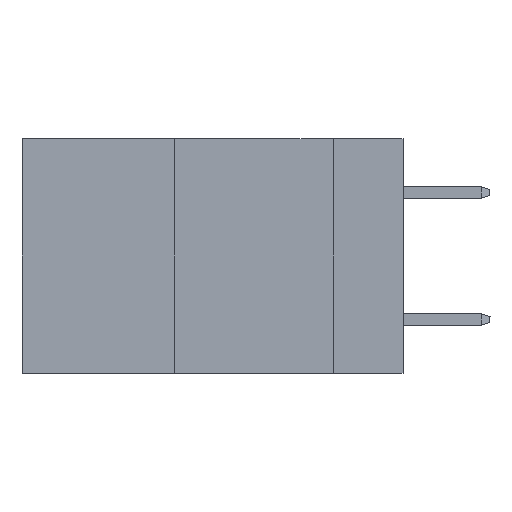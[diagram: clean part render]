
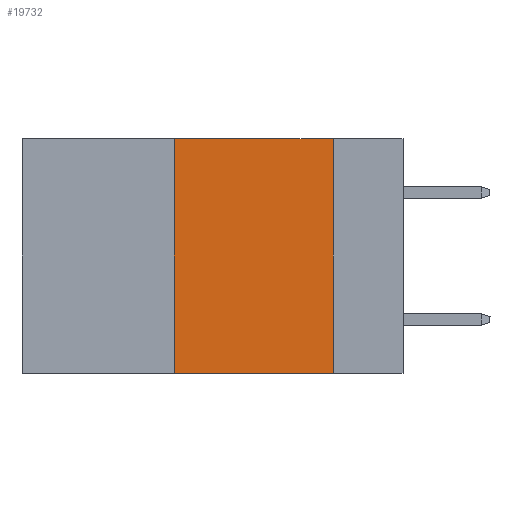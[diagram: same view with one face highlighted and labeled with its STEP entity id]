
A CAD part, left-side view. The second image highlights one B-rep face of the part: STEP entity #19732.
In plain terms, the highlighted planar face has unit normal (-1, 0, 0).
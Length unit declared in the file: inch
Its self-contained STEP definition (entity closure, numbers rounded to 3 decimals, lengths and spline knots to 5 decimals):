
#87 = EDGE_CURVE ( 'NONE', #24804, #4142, #3936, .T. ) ;
#2150 = DIRECTION ( 'NONE',  ( 0., 0., -1. ) ) ;
#3017 = LINE ( 'NONE', #14430, #6282 ) ;
#3355 = EDGE_CURVE ( 'NONE', #4142, #12133, #13696, .T. ) ;
#3687 = PLANE ( 'NONE',  #6561 ) ;
#3936 = LINE ( 'NONE', #23061, #21239 ) ;
#4142 = VERTEX_POINT ( 'NONE', #8129 ) ;
#4842 = CARTESIAN_POINT ( 'NONE',  ( 0., 0.36, 0. ) ) ;
#5101 = DIRECTION ( 'NONE',  ( 0., 0., -1. ) ) ;
#5926 = VECTOR ( 'NONE', #10092, 39.37008 ) ;
#6088 = EDGE_CURVE ( 'NONE', #7276, #24804, #16632, .T. ) ;
#6282 = VECTOR ( 'NONE', #14245, 39.37008 ) ;
#6561 = AXIS2_PLACEMENT_3D ( 'NONE', #15098, #18113, #2150 ) ;
#7276 = VERTEX_POINT ( 'NONE', #26984 ) ;
#7449 = CARTESIAN_POINT ( 'NONE',  ( 0., 0.11, -0.37 ) ) ;
#7567 = VECTOR ( 'NONE', #5101, 39.37008 ) ;
#8129 = CARTESIAN_POINT ( 'NONE',  ( 0., 0.11, 0. ) ) ;
#10092 = DIRECTION ( 'NONE',  ( 0., 0., 1. ) ) ;
#12133 = VERTEX_POINT ( 'NONE', #7449 ) ;
#12947 = ORIENTED_EDGE ( 'NONE', *, *, #87, .F. ) ;
#13214 = ORIENTED_EDGE ( 'NONE', *, *, #31818, .T. ) ;
#13696 = LINE ( 'NONE', #30988, #7567 ) ;
#14245 = DIRECTION ( 'NONE',  ( 0., -1., 0. ) ) ;
#14430 = CARTESIAN_POINT ( 'NONE',  ( 0., 0.6, -0.37 ) ) ;
#14837 = ORIENTED_EDGE ( 'NONE', *, *, #3355, .F. ) ;
#15098 = CARTESIAN_POINT ( 'NONE',  ( 0., 0.6, 0. ) ) ;
#15482 = EDGE_LOOP ( 'NONE', ( #14837, #12947, #26612, #13214 ) ) ;
#16632 = LINE ( 'NONE', #4842, #5926 ) ;
#18113 = DIRECTION ( 'NONE',  ( 1., 0., 0. ) ) ;
#19732 = ADVANCED_FACE ( 'NONE', ( #32387 ), #3687, .F. ) ;
#21239 = VECTOR ( 'NONE', #29257, 39.37008 ) ;
#23061 = CARTESIAN_POINT ( 'NONE',  ( 0., 0.6, 0. ) ) ;
#23396 = CARTESIAN_POINT ( 'NONE',  ( 0., 0.36, 0. ) ) ;
#24804 = VERTEX_POINT ( 'NONE', #23396 ) ;
#26612 = ORIENTED_EDGE ( 'NONE', *, *, #6088, .F. ) ;
#26984 = CARTESIAN_POINT ( 'NONE',  ( 0., 0.36, -0.37 ) ) ;
#29257 = DIRECTION ( 'NONE',  ( 0., -1., 0. ) ) ;
#30988 = CARTESIAN_POINT ( 'NONE',  ( 0., 0.11, 0. ) ) ;
#31818 = EDGE_CURVE ( 'NONE', #7276, #12133, #3017, .T. ) ;
#32387 = FACE_OUTER_BOUND ( 'NONE', #15482, .T. ) ;
